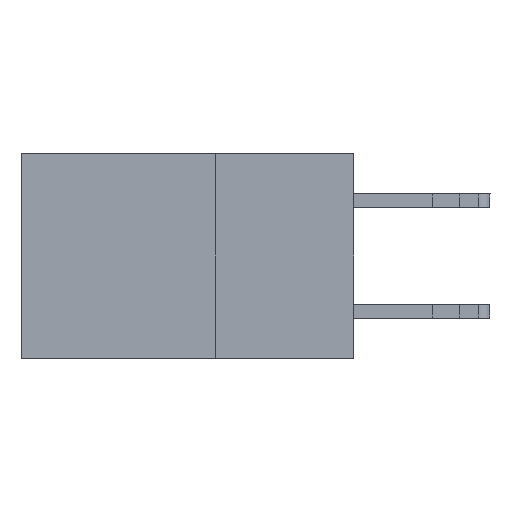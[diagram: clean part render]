
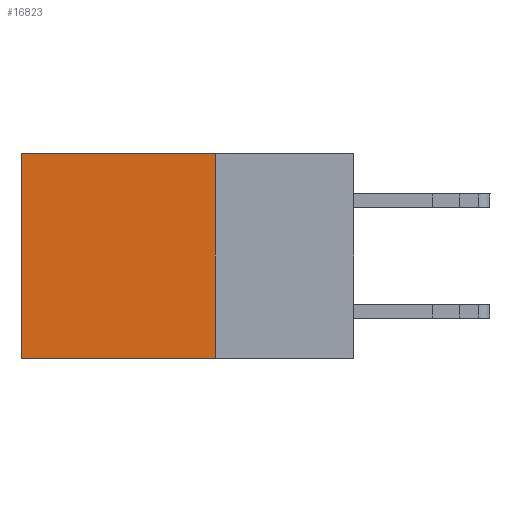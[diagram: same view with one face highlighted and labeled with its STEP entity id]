
A CAD part, left-side view. The second image highlights one B-rep face of the part: STEP entity #16823.
In plain terms, the highlighted planar face has unit normal (-1, 0, 0).
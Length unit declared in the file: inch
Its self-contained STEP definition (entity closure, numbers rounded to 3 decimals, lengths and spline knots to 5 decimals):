
#349 = VERTEX_POINT ( 'NONE', #6849 ) ;
#730 = CARTESIAN_POINT ( 'NONE',  ( 0.2875, 0.6, -0.37 ) ) ;
#899 = CARTESIAN_POINT ( 'NONE',  ( 0.2875, 0.6, 0. ) ) ;
#1075 = CARTESIAN_POINT ( 'NONE',  ( 0.2875, 0.25, -0.37 ) ) ;
#1368 = FACE_OUTER_BOUND ( 'NONE', #5109, .T. ) ;
#1984 = VECTOR ( 'NONE', #7110, 39.37008 ) ;
#2714 = ORIENTED_EDGE ( 'NONE', *, *, #11608, .F. ) ;
#2927 = PLANE ( 'NONE',  #8407 ) ;
#2996 = CARTESIAN_POINT ( 'NONE',  ( 0.2875, 0.25, 0. ) ) ;
#3288 = EDGE_CURVE ( 'NONE', #15348, #10314, #8913, .T. ) ;
#3567 = VERTEX_POINT ( 'NONE', #10031 ) ;
#5109 = EDGE_LOOP ( 'NONE', ( #13352, #10790, #2714, #16505 ) ) ;
#6849 = CARTESIAN_POINT ( 'NONE',  ( 0.2875, 0.25, 0. ) ) ;
#7110 = DIRECTION ( 'NONE',  ( 0., 0., -1. ) ) ;
#7222 = CARTESIAN_POINT ( 'NONE',  ( 0.2875, 0.25, -0.37 ) ) ;
#7227 = VECTOR ( 'NONE', #10047, 39.37008 ) ;
#7346 = LINE ( 'NONE', #899, #7227 ) ;
#8019 = CARTESIAN_POINT ( 'NONE',  ( 0.2875, 0.25, 0. ) ) ;
#8264 = EDGE_CURVE ( 'NONE', #3567, #10314, #7346, .T. ) ;
#8407 = AXIS2_PLACEMENT_3D ( 'NONE', #15798, #14505, #11898 ) ;
#8913 = LINE ( 'NONE', #1075, #10409 ) ;
#10031 = CARTESIAN_POINT ( 'NONE',  ( 0.2875, 0.6, 0. ) ) ;
#10047 = DIRECTION ( 'NONE',  ( 0., 0., -1. ) ) ;
#10314 = VERTEX_POINT ( 'NONE', #730 ) ;
#10328 = VECTOR ( 'NONE', #13314, 39.37008 ) ;
#10409 = VECTOR ( 'NONE', #11173, 39.37008 ) ;
#10790 = ORIENTED_EDGE ( 'NONE', *, *, #3288, .F. ) ;
#11095 = LINE ( 'NONE', #2996, #1984 ) ;
#11173 = DIRECTION ( 'NONE',  ( 0., 1., 0. ) ) ;
#11608 = EDGE_CURVE ( 'NONE', #349, #15348, #11095, .T. ) ;
#11898 = DIRECTION ( 'NONE',  ( 0., 0., -1. ) ) ;
#13234 = LINE ( 'NONE', #8019, #10328 ) ;
#13314 = DIRECTION ( 'NONE',  ( 0., 1., 0. ) ) ;
#13352 = ORIENTED_EDGE ( 'NONE', *, *, #8264, .T. ) ;
#14505 = DIRECTION ( 'NONE',  ( 1., 0., 0. ) ) ;
#15348 = VERTEX_POINT ( 'NONE', #7222 ) ;
#15798 = CARTESIAN_POINT ( 'NONE',  ( 0.2875, 0.25, 0. ) ) ;
#16480 = EDGE_CURVE ( 'NONE', #349, #3567, #13234, .T. ) ;
#16505 = ORIENTED_EDGE ( 'NONE', *, *, #16480, .T. ) ;
#16823 = ADVANCED_FACE ( 'NONE', ( #1368 ), #2927, .F. ) ;
